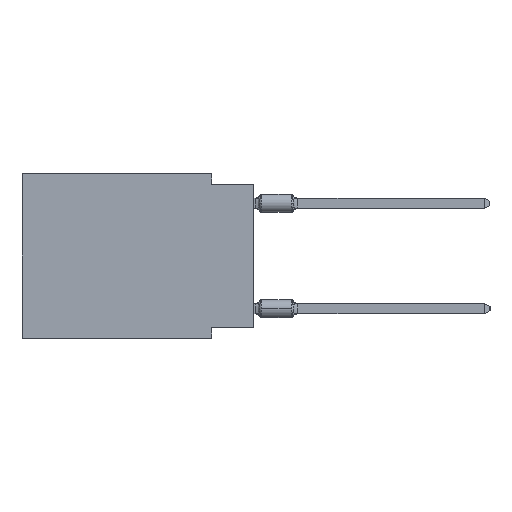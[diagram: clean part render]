
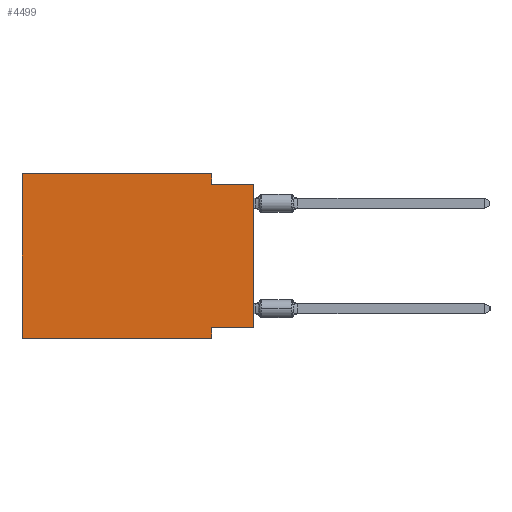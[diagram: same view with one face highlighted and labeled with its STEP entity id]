
A CAD part, left-side view. The second image highlights one B-rep face of the part: STEP entity #4499.
In plain terms, the highlighted planar face has unit normal (-1, 0, 0).
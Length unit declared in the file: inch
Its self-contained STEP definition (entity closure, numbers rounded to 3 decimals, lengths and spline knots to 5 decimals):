
#356 = DIRECTION ( 'NONE',  ( 0., 1., 0. ) ) ;
#1051 = LINE ( 'NONE', #34081, #3857 ) ;
#1279 = AXIS2_PLACEMENT_3D ( 'NONE', #9005, #22059, #18835 ) ;
#1658 = ORIENTED_EDGE ( 'NONE', *, *, #6655, .F. ) ;
#1914 = CARTESIAN_POINT ( 'NONE',  ( 0., 0.55, -0.39 ) ) ;
#2412 = ORIENTED_EDGE ( 'NONE', *, *, #31064, .T. ) ;
#3857 = VECTOR ( 'NONE', #40504, 39.37008 ) ;
#4006 = LINE ( 'NONE', #30401, #23792 ) ;
#4317 = ORIENTED_EDGE ( 'NONE', *, *, #15267, .F. ) ;
#4346 = CARTESIAN_POINT ( 'NONE',  ( 0., 0.1, 0. ) ) ;
#4499 = ADVANCED_FACE ( 'NONE', ( #12216 ), #38389, .F. ) ;
#4571 = CARTESIAN_POINT ( 'NONE',  ( 0., 0.55, -0.39 ) ) ;
#4839 = DIRECTION ( 'NONE',  ( 0., -1., 0. ) ) ;
#4878 = ORIENTED_EDGE ( 'NONE', *, *, #36091, .F. ) ;
#5171 = DIRECTION ( 'NONE',  ( 0., 0., 1. ) ) ;
#6574 = CARTESIAN_POINT ( 'NONE',  ( 0., 0.55, 0. ) ) ;
#6655 = EDGE_CURVE ( 'NONE', #31474, #13628, #36209, .T. ) ;
#6805 = DIRECTION ( 'NONE',  ( 0., 0., 1. ) ) ;
#7269 = LINE ( 'NONE', #17134, #26238 ) ;
#7573 = LINE ( 'NONE', #4571, #39568 ) ;
#8917 = EDGE_CURVE ( 'NONE', #36108, #16766, #16996, .T. ) ;
#9005 = CARTESIAN_POINT ( 'NONE',  ( 0., 0.55, 0. ) ) ;
#9190 = CARTESIAN_POINT ( 'NONE',  ( 0., 0.1, -0.025 ) ) ;
#9244 = ORIENTED_EDGE ( 'NONE', *, *, #33378, .F. ) ;
#12216 = FACE_OUTER_BOUND ( 'NONE', #40087, .T. ) ;
#13628 = VERTEX_POINT ( 'NONE', #6574 ) ;
#13702 = DIRECTION ( 'NONE',  ( 0., 0., -1. ) ) ;
#14525 = VERTEX_POINT ( 'NONE', #29962 ) ;
#15267 = EDGE_CURVE ( 'NONE', #13628, #36108, #1051, .T. ) ;
#16766 = VERTEX_POINT ( 'NONE', #9190 ) ;
#16996 = LINE ( 'NONE', #4346, #20034 ) ;
#17134 = CARTESIAN_POINT ( 'NONE',  ( 0., 0.1, -0.39 ) ) ;
#17414 = DIRECTION ( 'NONE',  ( 0., 0., -1. ) ) ;
#18835 = DIRECTION ( 'NONE',  ( 0., 0., -1. ) ) ;
#20007 = VECTOR ( 'NONE', #5171, 39.37008 ) ;
#20034 = VECTOR ( 'NONE', #17414, 39.37008 ) ;
#20165 = ORIENTED_EDGE ( 'NONE', *, *, #8917, .F. ) ;
#20847 = DIRECTION ( 'NONE',  ( 0., -1., 0. ) ) ;
#22059 = DIRECTION ( 'NONE',  ( 1., 0., 0. ) ) ;
#22401 = VERTEX_POINT ( 'NONE', #32097 ) ;
#22506 = EDGE_CURVE ( 'NONE', #31474, #22401, #7573, .T. ) ;
#23306 = EDGE_CURVE ( 'NONE', #16766, #39112, #4006, .T. ) ;
#23374 = ORIENTED_EDGE ( 'NONE', *, *, #22506, .T. ) ;
#23494 = CARTESIAN_POINT ( 'NONE',  ( 0., 0., -0.365 ) ) ;
#23792 = VECTOR ( 'NONE', #4839, 39.37008 ) ;
#24746 = VECTOR ( 'NONE', #6805, 39.37008 ) ;
#26238 = VECTOR ( 'NONE', #13702, 39.37008 ) ;
#27037 = VERTEX_POINT ( 'NONE', #33879 ) ;
#29962 = CARTESIAN_POINT ( 'NONE',  ( 0., 0.1, -0.365 ) ) ;
#30401 = CARTESIAN_POINT ( 'NONE',  ( 0., 0., -0.025 ) ) ;
#31064 = EDGE_CURVE ( 'NONE', #27037, #39112, #34581, .T. ) ;
#31146 = ORIENTED_EDGE ( 'NONE', *, *, #23306, .F. ) ;
#31474 = VERTEX_POINT ( 'NONE', #1914 ) ;
#32097 = CARTESIAN_POINT ( 'NONE',  ( 0., 0.1, -0.39 ) ) ;
#33378 = EDGE_CURVE ( 'NONE', #27037, #14525, #39399, .T. ) ;
#33431 = CARTESIAN_POINT ( 'NONE',  ( 0., 0.55, 0. ) ) ;
#33879 = CARTESIAN_POINT ( 'NONE',  ( 0., 0., -0.365 ) ) ;
#34081 = CARTESIAN_POINT ( 'NONE',  ( 0., 0.55, 0. ) ) ;
#34581 = LINE ( 'NONE', #40793, #20007 ) ;
#36091 = EDGE_CURVE ( 'NONE', #14525, #22401, #7269, .T. ) ;
#36108 = VERTEX_POINT ( 'NONE', #36885 ) ;
#36209 = LINE ( 'NONE', #33431, #24746 ) ;
#36885 = CARTESIAN_POINT ( 'NONE',  ( 0., 0.1, 0. ) ) ;
#38389 = PLANE ( 'NONE',  #1279 ) ;
#39112 = VERTEX_POINT ( 'NONE', #42223 ) ;
#39399 = LINE ( 'NONE', #23494, #40727 ) ;
#39568 = VECTOR ( 'NONE', #20847, 39.37008 ) ;
#40087 = EDGE_LOOP ( 'NONE', ( #2412, #31146, #20165, #4317, #1658, #23374, #4878, #9244 ) ) ;
#40504 = DIRECTION ( 'NONE',  ( 0., -1., 0. ) ) ;
#40727 = VECTOR ( 'NONE', #356, 39.37008 ) ;
#40793 = CARTESIAN_POINT ( 'NONE',  ( 0., 0., 0. ) ) ;
#42223 = CARTESIAN_POINT ( 'NONE',  ( 0., 0., -0.025 ) ) ;
